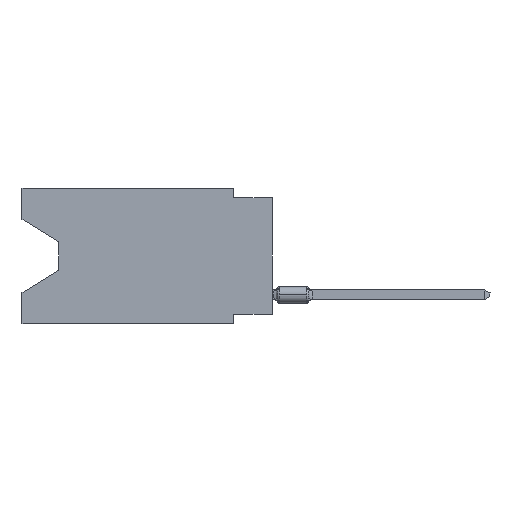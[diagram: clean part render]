
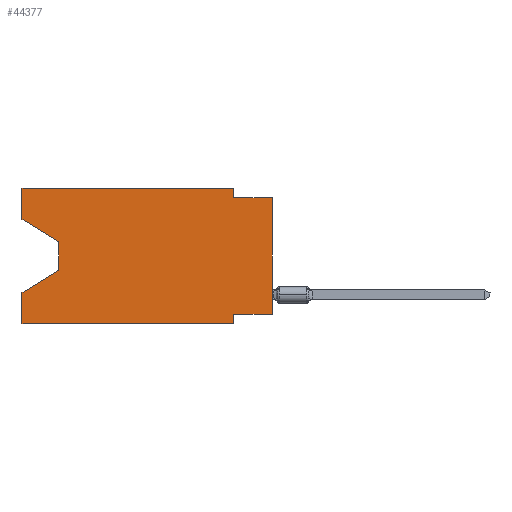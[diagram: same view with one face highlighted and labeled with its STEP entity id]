
A CAD part, left-side view. The second image highlights one B-rep face of the part: STEP entity #44377.
In plain terms, the highlighted planar face has unit normal (-1, 0, 0).
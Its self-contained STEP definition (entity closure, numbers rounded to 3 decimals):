
#282 = VECTOR ( 'NONE', #37411, 1000. ) ;
#556 = CARTESIAN_POINT ( 'NONE',  ( 0., 2.54, 0. ) ) ;
#1679 = ORIENTED_EDGE ( 'NONE', *, *, #13653, .F. ) ;
#1808 = EDGE_CURVE ( 'NONE', #3780, #35642, #44119, .T. ) ;
#2644 = ORIENTED_EDGE ( 'NONE', *, *, #31788, .T. ) ;
#3780 = VERTEX_POINT ( 'NONE', #54922 ) ;
#5841 = ORIENTED_EDGE ( 'NONE', *, *, #15555, .T. ) ;
#5892 = DIRECTION ( 'NONE',  ( 0., 0., -1. ) ) ;
#6555 = ORIENTED_EDGE ( 'NONE', *, *, #28332, .F. ) ;
#7178 = CARTESIAN_POINT ( 'NONE',  ( 0., 13.97, -5.385 ) ) ;
#8410 = LINE ( 'NONE', #7178, #68867 ) ;
#10843 = CARTESIAN_POINT ( 'NONE',  ( 0., 13.97, -3.505 ) ) ;
#11384 = ORIENTED_EDGE ( 'NONE', *, *, #29804, .F. ) ;
#13653 = EDGE_CURVE ( 'NONE', #23897, #55066, #77273, .T. ) ;
#15555 = EDGE_CURVE ( 'NONE', #23897, #53792, #20212, .T. ) ;
#16299 = LINE ( 'NONE', #10843, #65706 ) ;
#17574 = ORIENTED_EDGE ( 'NONE', *, *, #80440, .T. ) ;
#18207 = VECTOR ( 'NONE', #55375, 1000. ) ;
#19641 = EDGE_LOOP ( 'NONE', ( #5841, #17574, #56422, #48139, #24003, #11384, #6555, #2644, #25850, #72318, #56788, #1679 ) ) ;
#20212 = LINE ( 'NONE', #64732, #70578 ) ;
#20603 = CARTESIAN_POINT ( 'NONE',  ( 0., 13.97, -3.505 ) ) ;
#20734 = EDGE_CURVE ( 'NONE', #55066, #34822, #51002, .T. ) ;
#21334 = DIRECTION ( 'NONE',  ( 0., 1., 0. ) ) ;
#21624 = CARTESIAN_POINT ( 'NONE',  ( 0., 16.383, -2.038 ) ) ;
#23897 = VERTEX_POINT ( 'NONE', #21624 ) ;
#24003 = ORIENTED_EDGE ( 'NONE', *, *, #1808, .T. ) ;
#24292 = LINE ( 'NONE', #67972, #18207 ) ;
#25512 = CARTESIAN_POINT ( 'NONE',  ( 0., 2.54, 0. ) ) ;
#25850 = ORIENTED_EDGE ( 'NONE', *, *, #31891, .F. ) ;
#28305 = CARTESIAN_POINT ( 'NONE',  ( 0., 0., -0.635 ) ) ;
#28332 = EDGE_CURVE ( 'NONE', #67967, #71476, #53260, .T. ) ;
#28738 = DIRECTION ( 'NONE',  ( 1., 0., 0. ) ) ;
#29804 = EDGE_CURVE ( 'NONE', #71476, #35642, #31890, .T. ) ;
#30383 = FACE_OUTER_BOUND ( 'NONE', #19641, .T. ) ;
#31101 = CARTESIAN_POINT ( 'NONE',  ( 0., 16.383, -8.89 ) ) ;
#31165 = CARTESIAN_POINT ( 'NONE',  ( 0., 2.54, -8.89 ) ) ;
#31788 = EDGE_CURVE ( 'NONE', #67967, #70980, #35038, .T. ) ;
#31891 = EDGE_CURVE ( 'NONE', #69751, #70980, #45064, .T. ) ;
#31890 = LINE ( 'NONE', #64241, #57125 ) ;
#34822 = VERTEX_POINT ( 'NONE', #25512 ) ;
#35038 = LINE ( 'NONE', #36289, #61366 ) ;
#35186 = DIRECTION ( 'NONE',  ( 0., 0., -1. ) ) ;
#35642 = VERTEX_POINT ( 'NONE', #31165 ) ;
#36289 = CARTESIAN_POINT ( 'NONE',  ( 0., 0., 0. ) ) ;
#36716 = CARTESIAN_POINT ( 'NONE',  ( 0., 16.383, 0. ) ) ;
#37411 = DIRECTION ( 'NONE',  ( 0., -1., 0. ) ) ;
#38618 = CARTESIAN_POINT ( 'NONE',  ( 0., 16.383, 0. ) ) ;
#39127 = LINE ( 'NONE', #556, #67136 ) ;
#40648 = CARTESIAN_POINT ( 'NONE',  ( 0., 0., -8.255 ) ) ;
#42391 = CARTESIAN_POINT ( 'NONE',  ( 0., 13.97, -5.385 ) ) ;
#43551 = VECTOR ( 'NONE', #21334, 1000. ) ;
#43817 = CARTESIAN_POINT ( 'NONE',  ( 0., 0., -0.635 ) ) ;
#44119 = LINE ( 'NONE', #31101, #282 ) ;
#44377 = ADVANCED_FACE ( 'NONE', ( #30383 ), #80388, .F. ) ;
#44986 = EDGE_CURVE ( 'NONE', #82645, #49857, #8410, .T. ) ;
#45064 = LINE ( 'NONE', #43817, #65442 ) ;
#47429 = EDGE_CURVE ( 'NONE', #3780, #49857, #24292, .T. ) ;
#48139 = ORIENTED_EDGE ( 'NONE', *, *, #47429, .F. ) ;
#48873 = VECTOR ( 'NONE', #64255, 1000. ) ;
#49857 = VERTEX_POINT ( 'NONE', #82669 ) ;
#51002 = LINE ( 'NONE', #36716, #52229 ) ;
#52098 = DIRECTION ( 'NONE',  ( 0., 0.855, -0.519 ) ) ;
#52229 = VECTOR ( 'NONE', #56049, 1000. ) ;
#53260 = LINE ( 'NONE', #40648, #43551 ) ;
#53792 = VERTEX_POINT ( 'NONE', #20603 ) ;
#54922 = CARTESIAN_POINT ( 'NONE',  ( 0., 16.383, -8.89 ) ) ;
#55066 = VERTEX_POINT ( 'NONE', #68081 ) ;
#55375 = DIRECTION ( 'NONE',  ( 0., 0., 1. ) ) ;
#55591 = DIRECTION ( 'NONE',  ( 0., 0., -1. ) ) ;
#56049 = DIRECTION ( 'NONE',  ( 0., -1., 0. ) ) ;
#56422 = ORIENTED_EDGE ( 'NONE', *, *, #44986, .T. ) ;
#56788 = ORIENTED_EDGE ( 'NONE', *, *, #20734, .F. ) ;
#57125 = VECTOR ( 'NONE', #5892, 1000. ) ;
#58466 = DIRECTION ( 'NONE',  ( 0., 0., -1. ) ) ;
#59348 = AXIS2_PLACEMENT_3D ( 'NONE', #60655, #28738, #55591 ) ;
#60190 = CARTESIAN_POINT ( 'NONE',  ( 0., 0., -8.255 ) ) ;
#60655 = CARTESIAN_POINT ( 'NONE',  ( 0., 16.383, 0. ) ) ;
#61366 = VECTOR ( 'NONE', #79985, 1000. ) ;
#63142 = EDGE_CURVE ( 'NONE', #34822, #69751, #39127, .T. ) ;
#64241 = CARTESIAN_POINT ( 'NONE',  ( 0., 2.54, -8.89 ) ) ;
#64255 = DIRECTION ( 'NONE',  ( 0., 0., 1. ) ) ;
#64732 = CARTESIAN_POINT ( 'NONE',  ( 0., 16.383, -2.038 ) ) ;
#65136 = DIRECTION ( 'NONE',  ( 0., -0.855, -0.519 ) ) ;
#65442 = VECTOR ( 'NONE', #69459, 1000. ) ;
#65706 = VECTOR ( 'NONE', #35186, 1000. ) ;
#67136 = VECTOR ( 'NONE', #58466, 1000. ) ;
#67967 = VERTEX_POINT ( 'NONE', #60190 ) ;
#67972 = CARTESIAN_POINT ( 'NONE',  ( 0., 16.383, 0. ) ) ;
#68081 = CARTESIAN_POINT ( 'NONE',  ( 0., 16.383, 0. ) ) ;
#68867 = VECTOR ( 'NONE', #52098, 1000. ) ;
#69312 = CARTESIAN_POINT ( 'NONE',  ( 0., 2.54, -0.635 ) ) ;
#69459 = DIRECTION ( 'NONE',  ( 0., -1., 0. ) ) ;
#69751 = VERTEX_POINT ( 'NONE', #69312 ) ;
#70578 = VECTOR ( 'NONE', #65136, 1000. ) ;
#70980 = VERTEX_POINT ( 'NONE', #28305 ) ;
#71476 = VERTEX_POINT ( 'NONE', #79852 ) ;
#72318 = ORIENTED_EDGE ( 'NONE', *, *, #63142, .F. ) ;
#77273 = LINE ( 'NONE', #38618, #48873 ) ;
#79852 = CARTESIAN_POINT ( 'NONE',  ( 0., 2.54, -8.255 ) ) ;
#79985 = DIRECTION ( 'NONE',  ( 0., 0., 1. ) ) ;
#80388 = PLANE ( 'NONE',  #59348 ) ;
#80440 = EDGE_CURVE ( 'NONE', #53792, #82645, #16299, .T. ) ;
#82645 = VERTEX_POINT ( 'NONE', #42391 ) ;
#82669 = CARTESIAN_POINT ( 'NONE',  ( 0., 16.383, -6.852 ) ) ;
